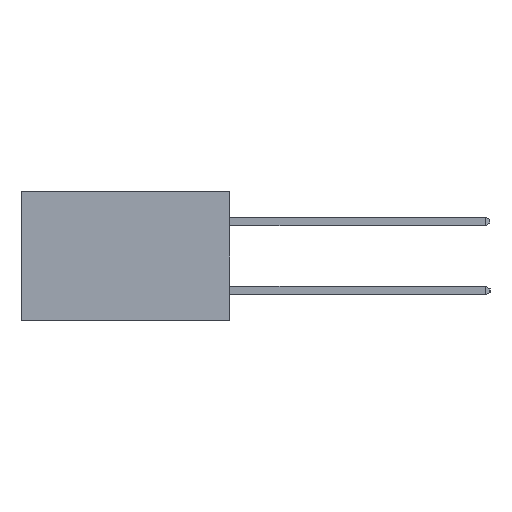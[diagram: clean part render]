
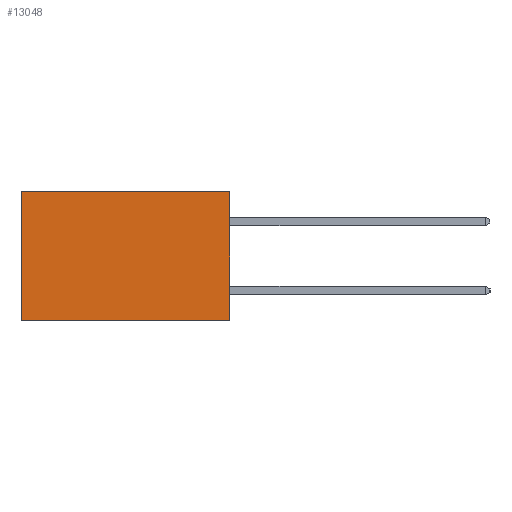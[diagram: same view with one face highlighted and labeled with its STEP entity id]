
A CAD part, left-side view. The second image highlights one B-rep face of the part: STEP entity #13048.
In plain terms, the highlighted planar face has unit normal (-1, 0, 0).
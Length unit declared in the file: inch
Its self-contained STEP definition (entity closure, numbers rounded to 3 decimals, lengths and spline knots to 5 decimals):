
#556 = VERTEX_POINT ( 'NONE', #3706 ) ;
#621 = PLANE ( 'NONE',  #6874 ) ;
#927 = LINE ( 'NONE', #9077, #1302 ) ;
#1059 = VECTOR ( 'NONE', #6931, 39.37008 ) ;
#1302 = VECTOR ( 'NONE', #1625, 39.37008 ) ;
#1520 = CARTESIAN_POINT ( 'NONE',  ( 0.2615, 0.6, 0. ) ) ;
#1625 = DIRECTION ( 'NONE',  ( 0., 1., 0. ) ) ;
#2265 = EDGE_CURVE ( 'NONE', #6577, #8626, #8095, .T. ) ;
#3186 = DIRECTION ( 'NONE',  ( 0., 0., -1. ) ) ;
#3663 = VERTEX_POINT ( 'NONE', #15378 ) ;
#3706 = CARTESIAN_POINT ( 'NONE',  ( 0.2615, 0., -0.37 ) ) ;
#4260 = CARTESIAN_POINT ( 'NONE',  ( 0.2615, 0.6, -0.37 ) ) ;
#4590 = ORIENTED_EDGE ( 'NONE', *, *, #15360, .F. ) ;
#4883 = VECTOR ( 'NONE', #11997, 39.37008 ) ;
#5058 = EDGE_LOOP ( 'NONE', ( #9857, #4590, #5662, #13656 ) ) ;
#5662 = ORIENTED_EDGE ( 'NONE', *, *, #11769, .F. ) ;
#6222 = VECTOR ( 'NONE', #13581, 39.37008 ) ;
#6577 = VERTEX_POINT ( 'NONE', #1520 ) ;
#6874 = AXIS2_PLACEMENT_3D ( 'NONE', #9329, #10525, #3186 ) ;
#6931 = DIRECTION ( 'NONE',  ( 0., 0., -1. ) ) ;
#8095 = LINE ( 'NONE', #10076, #4883 ) ;
#8489 = LINE ( 'NONE', #11696, #1059 ) ;
#8626 = VERTEX_POINT ( 'NONE', #4260 ) ;
#9077 = CARTESIAN_POINT ( 'NONE',  ( 0.2615, 0., 0. ) ) ;
#9329 = CARTESIAN_POINT ( 'NONE',  ( 0.2615, 0., -0.37 ) ) ;
#9857 = ORIENTED_EDGE ( 'NONE', *, *, #2265, .T. ) ;
#10076 = CARTESIAN_POINT ( 'NONE',  ( 0.2615, 0.6, -0.37 ) ) ;
#10525 = DIRECTION ( 'NONE',  ( 1., 0., 0. ) ) ;
#11215 = CARTESIAN_POINT ( 'NONE',  ( 0.2615, 0., -0.37 ) ) ;
#11696 = CARTESIAN_POINT ( 'NONE',  ( 0.2615, 0., -0.37 ) ) ;
#11769 = EDGE_CURVE ( 'NONE', #3663, #556, #8489, .T. ) ;
#11997 = DIRECTION ( 'NONE',  ( 0., 0., -1. ) ) ;
#12564 = LINE ( 'NONE', #11215, #6222 ) ;
#13048 = ADVANCED_FACE ( 'NONE', ( #14734 ), #621, .F. ) ;
#13581 = DIRECTION ( 'NONE',  ( 0., 1., 0. ) ) ;
#13656 = ORIENTED_EDGE ( 'NONE', *, *, #14243, .T. ) ;
#14243 = EDGE_CURVE ( 'NONE', #3663, #6577, #927, .T. ) ;
#14734 = FACE_OUTER_BOUND ( 'NONE', #5058, .T. ) ;
#15360 = EDGE_CURVE ( 'NONE', #556, #8626, #12564, .T. ) ;
#15378 = CARTESIAN_POINT ( 'NONE',  ( 0.2615, 0., 0. ) ) ;
